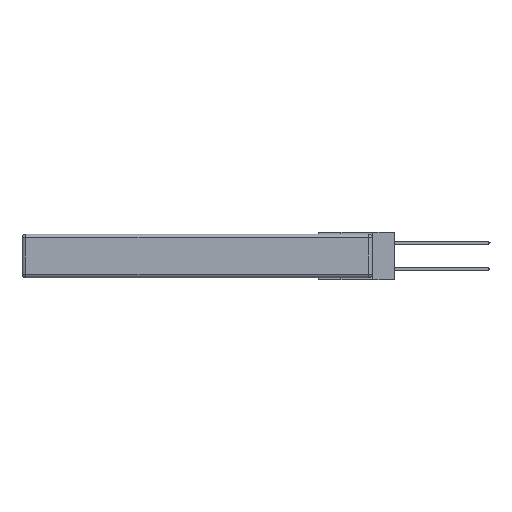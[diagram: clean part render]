
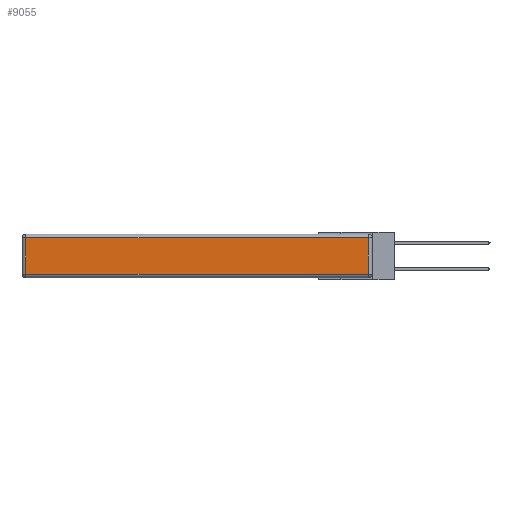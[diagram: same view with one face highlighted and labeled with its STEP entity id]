
A CAD part, left-side view. The second image highlights one B-rep face of the part: STEP entity #9055.
In plain terms, the highlighted planar face has unit normal (-1, 0, 0).
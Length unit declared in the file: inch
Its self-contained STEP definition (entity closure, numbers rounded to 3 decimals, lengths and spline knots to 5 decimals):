
#155 = ORIENTED_EDGE ( 'NONE', *, *, #613, .T. ) ;
#613 = EDGE_CURVE ( 'NONE', #9176, #6489, #5723, .T. ) ;
#906 = CARTESIAN_POINT ( 'NONE',  ( 0., 2.72, -0.313 ) ) ;
#1267 = DIRECTION ( 'NONE',  ( 0., 1., 0. ) ) ;
#1733 = DIRECTION ( 'NONE',  ( 0., 0., 1. ) ) ;
#1764 = DIRECTION ( 'NONE',  ( 0., 0., -1. ) ) ;
#2023 = LINE ( 'NONE', #2805, #6583 ) ;
#2044 = PLANE ( 'NONE',  #9507 ) ;
#2406 = CARTESIAN_POINT ( 'NONE',  ( 0., 2.75, -0.03 ) ) ;
#2505 = CARTESIAN_POINT ( 'NONE',  ( 0., 2.72, -0.03 ) ) ;
#2805 = CARTESIAN_POINT ( 'NONE',  ( 0., 0.03, -0.343 ) ) ;
#3066 = ORIENTED_EDGE ( 'NONE', *, *, #5722, .T. ) ;
#3235 = VECTOR ( 'NONE', #5195, 39.37008 ) ;
#4047 = CARTESIAN_POINT ( 'NONE',  ( 0., 2.72, -0.343 ) ) ;
#5195 = DIRECTION ( 'NONE',  ( 0., -1., 0. ) ) ;
#5272 = CARTESIAN_POINT ( 'NONE',  ( 0., 0., -0.343 ) ) ;
#5299 = EDGE_LOOP ( 'NONE', ( #12966, #13617, #155, #3066 ) ) ;
#5318 = EDGE_CURVE ( 'NONE', #11177, #9176, #2023, .T. ) ;
#5722 = EDGE_CURVE ( 'NONE', #6489, #11199, #8695, .T. ) ;
#5723 = LINE ( 'NONE', #2406, #12122 ) ;
#5784 = EDGE_CURVE ( 'NONE', #11199, #11177, #7628, .T. ) ;
#6489 = VERTEX_POINT ( 'NONE', #2505 ) ;
#6553 = DIRECTION ( 'NONE',  ( -1., 0., 0. ) ) ;
#6583 = VECTOR ( 'NONE', #1733, 39.37008 ) ;
#7628 = LINE ( 'NONE', #12001, #3235 ) ;
#8160 = FACE_OUTER_BOUND ( 'NONE', #5299, .T. ) ;
#8695 = LINE ( 'NONE', #4047, #9051 ) ;
#9051 = VECTOR ( 'NONE', #1764, 39.37008 ) ;
#9055 = ADVANCED_FACE ( 'NONE', ( #8160 ), #2044, .T. ) ;
#9176 = VERTEX_POINT ( 'NONE', #9654 ) ;
#9388 = CARTESIAN_POINT ( 'NONE',  ( 0., 0.03, -0.313 ) ) ;
#9507 = AXIS2_PLACEMENT_3D ( 'NONE', #5272, #6553, #14309 ) ;
#9654 = CARTESIAN_POINT ( 'NONE',  ( 0., 0.03, -0.03 ) ) ;
#11177 = VERTEX_POINT ( 'NONE', #9388 ) ;
#11199 = VERTEX_POINT ( 'NONE', #906 ) ;
#12001 = CARTESIAN_POINT ( 'NONE',  ( 0., 0., -0.313 ) ) ;
#12122 = VECTOR ( 'NONE', #1267, 39.37008 ) ;
#12966 = ORIENTED_EDGE ( 'NONE', *, *, #5784, .T. ) ;
#13617 = ORIENTED_EDGE ( 'NONE', *, *, #5318, .T. ) ;
#14309 = DIRECTION ( 'NONE',  ( 0., 0., 1. ) ) ;
